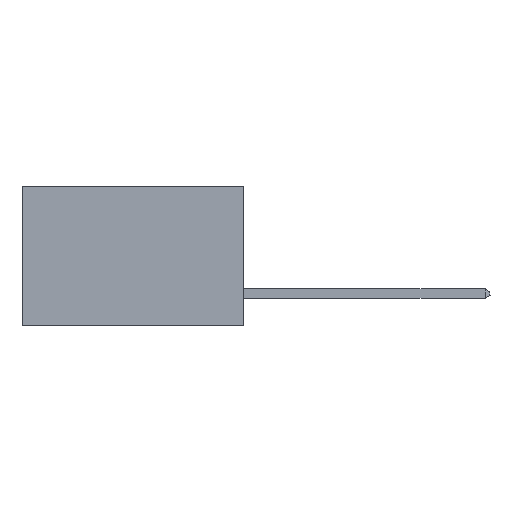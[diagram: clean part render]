
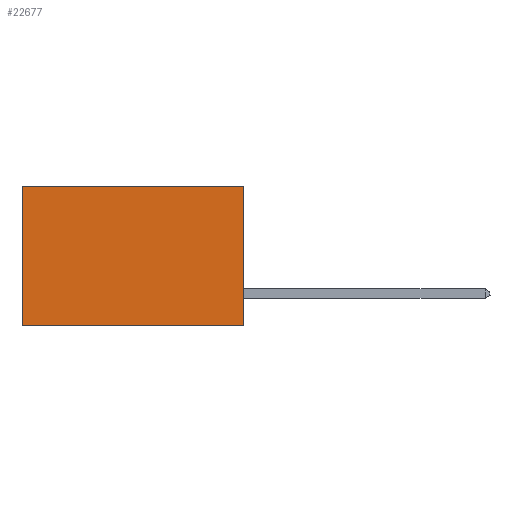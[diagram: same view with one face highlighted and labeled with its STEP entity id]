
A CAD part, left-side view. The second image highlights one B-rep face of the part: STEP entity #22677.
In plain terms, the highlighted planar face has unit normal (-1, 0, 0).
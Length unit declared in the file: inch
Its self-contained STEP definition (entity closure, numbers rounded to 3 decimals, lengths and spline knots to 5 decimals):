
#1358 = EDGE_CURVE ( 'NONE', #22430, #22798, #24051, .T. ) ;
#2879 = VERTEX_POINT ( 'NONE', #5709 ) ;
#2944 = ORIENTED_EDGE ( 'NONE', *, *, #9717, .T. ) ;
#3410 = FACE_OUTER_BOUND ( 'NONE', #17664, .T. ) ;
#3750 = CARTESIAN_POINT ( 'NONE',  ( 0.277, 0., -0.37 ) ) ;
#3777 = LINE ( 'NONE', #3750, #14393 ) ;
#4073 = VERTEX_POINT ( 'NONE', #8865 ) ;
#4498 = DIRECTION ( 'NONE',  ( 1., 0., 0. ) ) ;
#5709 = CARTESIAN_POINT ( 'NONE',  ( 0.277, 0.59, 0. ) ) ;
#6354 = CARTESIAN_POINT ( 'NONE',  ( 0.277, 0., -0.37 ) ) ;
#6596 = DIRECTION ( 'NONE',  ( 0., 0., -1. ) ) ;
#6742 = AXIS2_PLACEMENT_3D ( 'NONE', #13887, #4498, #17625 ) ;
#8670 = ORIENTED_EDGE ( 'NONE', *, *, #10876, .F. ) ;
#8865 = CARTESIAN_POINT ( 'NONE',  ( 0.277, 0.59, -0.37 ) ) ;
#9344 = CARTESIAN_POINT ( 'NONE',  ( 0.277, 0., 0. ) ) ;
#9717 = EDGE_CURVE ( 'NONE', #22430, #2879, #15589, .T. ) ;
#10186 = CARTESIAN_POINT ( 'NONE',  ( 0.277, 0.59, -0.37 ) ) ;
#10617 = EDGE_CURVE ( 'NONE', #2879, #4073, #14701, .T. ) ;
#10876 = EDGE_CURVE ( 'NONE', #22798, #4073, #3777, .T. ) ;
#11491 = DIRECTION ( 'NONE',  ( 0., 1., 0. ) ) ;
#13887 = CARTESIAN_POINT ( 'NONE',  ( 0.277, 0., -0.37 ) ) ;
#14393 = VECTOR ( 'NONE', #16899, 39.37008 ) ;
#14701 = LINE ( 'NONE', #10186, #20262 ) ;
#14998 = VECTOR ( 'NONE', #11491, 39.37008 ) ;
#15589 = LINE ( 'NONE', #20823, #14998 ) ;
#15757 = PLANE ( 'NONE',  #6742 ) ;
#16899 = DIRECTION ( 'NONE',  ( 0., 1., 0. ) ) ;
#17625 = DIRECTION ( 'NONE',  ( 0., 0., -1. ) ) ;
#17664 = EDGE_LOOP ( 'NONE', ( #24269, #8670, #21728, #2944 ) ) ;
#19328 = VECTOR ( 'NONE', #6596, 39.37008 ) ;
#20262 = VECTOR ( 'NONE', #23302, 39.37008 ) ;
#20823 = CARTESIAN_POINT ( 'NONE',  ( 0.277, 0., 0. ) ) ;
#21657 = CARTESIAN_POINT ( 'NONE',  ( 0.277, 0., -0.37 ) ) ;
#21728 = ORIENTED_EDGE ( 'NONE', *, *, #1358, .F. ) ;
#22430 = VERTEX_POINT ( 'NONE', #9344 ) ;
#22677 = ADVANCED_FACE ( 'NONE', ( #3410 ), #15757, .F. ) ;
#22798 = VERTEX_POINT ( 'NONE', #21657 ) ;
#23302 = DIRECTION ( 'NONE',  ( 0., 0., -1. ) ) ;
#24051 = LINE ( 'NONE', #6354, #19328 ) ;
#24269 = ORIENTED_EDGE ( 'NONE', *, *, #10617, .T. ) ;
